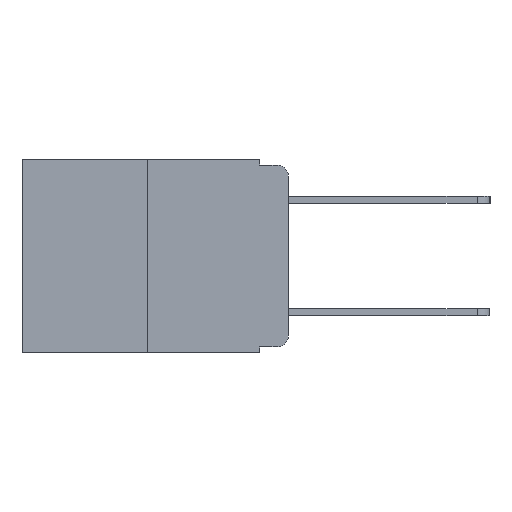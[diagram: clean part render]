
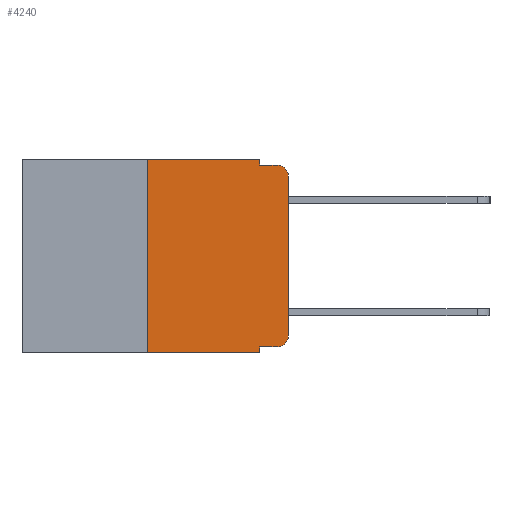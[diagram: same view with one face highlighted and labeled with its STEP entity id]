
A CAD part, left-side view. The second image highlights one B-rep face of the part: STEP entity #4240.
In plain terms, the highlighted planar face has unit normal (-1, 0, 0).
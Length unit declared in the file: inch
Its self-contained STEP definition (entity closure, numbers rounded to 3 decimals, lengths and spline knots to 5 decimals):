
#130 = VECTOR ( 'NONE', #11889, 39.37008 ) ;
#259 = CARTESIAN_POINT ( 'NONE',  ( 0., 0., -0.03 ) ) ;
#287 = VERTEX_POINT ( 'NONE', #10640 ) ;
#367 = VECTOR ( 'NONE', #9783, 39.37008 ) ;
#373 = EDGE_CURVE ( 'NONE', #6576, #8388, #3497, .T. ) ;
#450 = CARTESIAN_POINT ( 'NONE',  ( 0., 0., 0. ) ) ;
#581 = FACE_OUTER_BOUND ( 'NONE', #8595, .T. ) ;
#807 = DIRECTION ( 'NONE',  ( 1., 0., 0. ) ) ;
#1200 = VECTOR ( 'NONE', #9520, 39.37008 ) ;
#1835 = EDGE_CURVE ( 'NONE', #12787, #7315, #11682, .T. ) ;
#1922 = ORIENTED_EDGE ( 'NONE', *, *, #1835, .T. ) ;
#2543 = CARTESIAN_POINT ( 'NONE',  ( 0., 0.051, 0. ) ) ;
#2556 = LINE ( 'NONE', #7894, #367 ) ;
#2715 = EDGE_CURVE ( 'NONE', #7315, #8817, #9412, .T. ) ;
#2784 = DIRECTION ( 'NONE',  ( 0., -1., 0. ) ) ;
#3065 = ORIENTED_EDGE ( 'NONE', *, *, #12011, .F. ) ;
#3228 = LINE ( 'NONE', #2543, #8417 ) ;
#3259 = LINE ( 'NONE', #12245, #10866 ) ;
#3346 = ORIENTED_EDGE ( 'NONE', *, *, #373, .F. ) ;
#3433 = ORIENTED_EDGE ( 'NONE', *, *, #12564, .F. ) ;
#3495 = ORIENTED_EDGE ( 'NONE', *, *, #11440, .F. ) ;
#3497 = LINE ( 'NONE', #11106, #8644 ) ;
#3591 = ORIENTED_EDGE ( 'NONE', *, *, #4137, .T. ) ;
#3608 = ORIENTED_EDGE ( 'NONE', *, *, #10813, .F. ) ;
#3693 = ORIENTED_EDGE ( 'NONE', *, *, #2715, .T. ) ;
#3781 = ORIENTED_EDGE ( 'NONE', *, *, #10229, .T. ) ;
#3796 = ORIENTED_EDGE ( 'NONE', *, *, #9006, .T. ) ;
#4137 = EDGE_CURVE ( 'NONE', #4395, #5581, #3259, .T. ) ;
#4240 = ADVANCED_FACE ( 'NONE', ( #581 ), #6180, .F. ) ;
#4395 = VERTEX_POINT ( 'NONE', #12643 ) ;
#4554 = DIRECTION ( 'NONE',  ( -1., 0., 0. ) ) ;
#5045 = CARTESIAN_POINT ( 'NONE',  ( 0., 0.02, -0.03 ) ) ;
#5581 = VERTEX_POINT ( 'NONE', #10494 ) ;
#5674 = DIRECTION ( 'NONE',  ( -1., 0., 0. ) ) ;
#5870 = CARTESIAN_POINT ( 'NONE',  ( 0., 0.051, -0.01 ) ) ;
#6180 = PLANE ( 'NONE',  #8877 ) ;
#6227 = LINE ( 'NONE', #11010, #130 ) ;
#6549 = AXIS2_PLACEMENT_3D ( 'NONE', #5045, #5674, #10037 ) ;
#6576 = VERTEX_POINT ( 'NONE', #7103 ) ;
#6688 = VERTEX_POINT ( 'NONE', #10193 ) ;
#6899 = DIRECTION ( 'NONE',  ( 0., 0., 1. ) ) ;
#7103 = CARTESIAN_POINT ( 'NONE',  ( 0., 0.051, 0. ) ) ;
#7183 = CARTESIAN_POINT ( 'NONE',  ( 0., 0.473, 0. ) ) ;
#7315 = VERTEX_POINT ( 'NONE', #259 ) ;
#7894 = CARTESIAN_POINT ( 'NONE',  ( 0., 0.25, 0. ) ) ;
#7995 = VERTEX_POINT ( 'NONE', #9255 ) ;
#8159 = DIRECTION ( 'NONE',  ( 0., 0., -1. ) ) ;
#8388 = VERTEX_POINT ( 'NONE', #5870 ) ;
#8417 = VECTOR ( 'NONE', #12371, 39.37008 ) ;
#8595 = EDGE_LOOP ( 'NONE', ( #1922, #3693, #3065, #3346, #3433, #3495, #3591, #3608, #3781, #3796 ) ) ;
#8611 = CARTESIAN_POINT ( 'NONE',  ( 0., 0.051, -0.01 ) ) ;
#8644 = VECTOR ( 'NONE', #11585, 39.37008 ) ;
#8817 = VERTEX_POINT ( 'NONE', #10137 ) ;
#8877 = AXIS2_PLACEMENT_3D ( 'NONE', #7183, #807, #8159 ) ;
#9006 = EDGE_CURVE ( 'NONE', #7995, #12787, #12370, .T. ) ;
#9255 = CARTESIAN_POINT ( 'NONE',  ( 0., 0.02, -0.333 ) ) ;
#9290 = VECTOR ( 'NONE', #6899, 39.37008 ) ;
#9311 = VECTOR ( 'NONE', #2784, 39.37008 ) ;
#9409 = LINE ( 'NONE', #8611, #1200 ) ;
#9412 = CIRCLE ( 'NONE', #6549, 0.02 ) ;
#9520 = DIRECTION ( 'NONE',  ( 0., -1., 0. ) ) ;
#9783 = DIRECTION ( 'NONE',  ( 0., 0., 1. ) ) ;
#9905 = LINE ( 'NONE', #11677, #9311 ) ;
#10037 = DIRECTION ( 'NONE',  ( 0., 0., -1. ) ) ;
#10087 = AXIS2_PLACEMENT_3D ( 'NONE', #10405, #4554, #11316 ) ;
#10137 = CARTESIAN_POINT ( 'NONE',  ( 0., 0.02, -0.01 ) ) ;
#10193 = CARTESIAN_POINT ( 'NONE',  ( 0., 0.25, 0. ) ) ;
#10229 = EDGE_CURVE ( 'NONE', #287, #7995, #9905, .T. ) ;
#10405 = CARTESIAN_POINT ( 'NONE',  ( 0., 0.02, -0.313 ) ) ;
#10494 = CARTESIAN_POINT ( 'NONE',  ( 0., 0.051, -0.343 ) ) ;
#10640 = CARTESIAN_POINT ( 'NONE',  ( 0., 0.051, -0.333 ) ) ;
#10813 = EDGE_CURVE ( 'NONE', #287, #5581, #3228, .T. ) ;
#10866 = VECTOR ( 'NONE', #12291, 39.37008 ) ;
#11010 = CARTESIAN_POINT ( 'NONE',  ( 0., 0.473, 0. ) ) ;
#11106 = CARTESIAN_POINT ( 'NONE',  ( 0., 0.051, 0. ) ) ;
#11316 = DIRECTION ( 'NONE',  ( 0., 0., -1. ) ) ;
#11440 = EDGE_CURVE ( 'NONE', #4395, #6688, #2556, .T. ) ;
#11585 = DIRECTION ( 'NONE',  ( 0., 0., -1. ) ) ;
#11677 = CARTESIAN_POINT ( 'NONE',  ( 0., 0.051, -0.333 ) ) ;
#11682 = LINE ( 'NONE', #450, #9290 ) ;
#11889 = DIRECTION ( 'NONE',  ( 0., -1., 0. ) ) ;
#12011 = EDGE_CURVE ( 'NONE', #8388, #8817, #9409, .T. ) ;
#12134 = CARTESIAN_POINT ( 'NONE',  ( 0., 0., -0.313 ) ) ;
#12245 = CARTESIAN_POINT ( 'NONE',  ( 0., 0.473, -0.343 ) ) ;
#12291 = DIRECTION ( 'NONE',  ( 0., -1., 0. ) ) ;
#12370 = CIRCLE ( 'NONE', #10087, 0.02 ) ;
#12371 = DIRECTION ( 'NONE',  ( 0., 0., -1. ) ) ;
#12564 = EDGE_CURVE ( 'NONE', #6688, #6576, #6227, .T. ) ;
#12643 = CARTESIAN_POINT ( 'NONE',  ( 0., 0.25, -0.343 ) ) ;
#12787 = VERTEX_POINT ( 'NONE', #12134 ) ;
